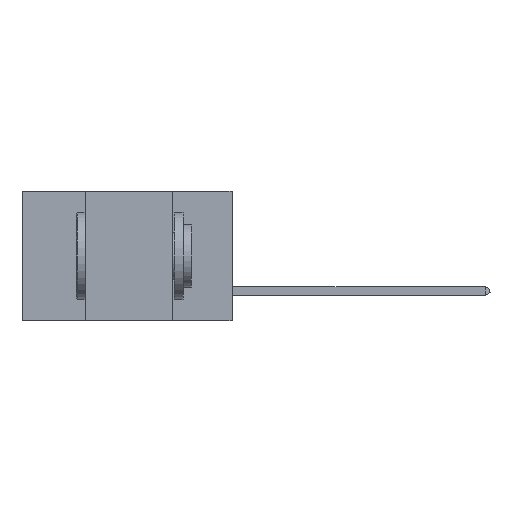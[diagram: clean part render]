
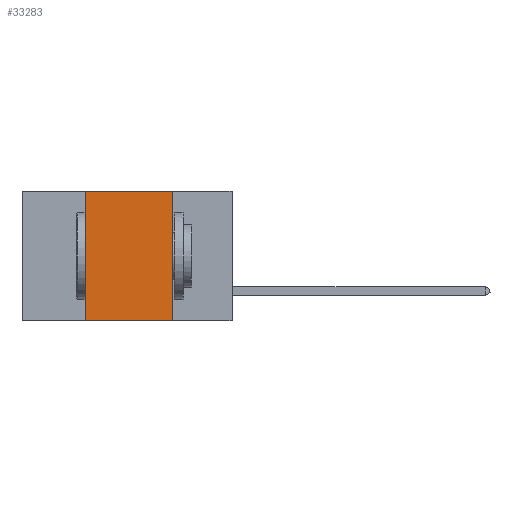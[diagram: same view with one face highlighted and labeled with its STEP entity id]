
A CAD part, left-side view. The second image highlights one B-rep face of the part: STEP entity #33283.
In plain terms, the highlighted planar face has unit normal (-1, 0, 0).
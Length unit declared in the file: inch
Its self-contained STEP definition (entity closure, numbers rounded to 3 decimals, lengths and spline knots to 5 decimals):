
#28 = VERTEX_POINT ( 'NONE', #24988 ) ;
#53 = ORIENTED_EDGE ( 'NONE', *, *, #757, .F. ) ;
#757 = EDGE_CURVE ( 'NONE', #8584, #9628, #33782, .T. ) ;
#4988 = PLANE ( 'NONE',  #29335 ) ;
#8259 = CARTESIAN_POINT ( 'NONE',  ( 0., 0.6, 0. ) ) ;
#8584 = VERTEX_POINT ( 'NONE', #9496 ) ;
#9496 = CARTESIAN_POINT ( 'NONE',  ( 0., 0.42, -0.37 ) ) ;
#9628 = VERTEX_POINT ( 'NONE', #25526 ) ;
#9767 = LINE ( 'NONE', #38687, #16532 ) ;
#12435 = ORIENTED_EDGE ( 'NONE', *, *, #34572, .F. ) ;
#12849 = DIRECTION ( 'NONE',  ( 0., 0., -1. ) ) ;
#13014 = CARTESIAN_POINT ( 'NONE',  ( 0., 0.17, 0. ) ) ;
#13269 = FACE_OUTER_BOUND ( 'NONE', #18787, .T. ) ;
#14413 = VERTEX_POINT ( 'NONE', #37573 ) ;
#15371 = DIRECTION ( 'NONE',  ( 0., 0., -1. ) ) ;
#16532 = VECTOR ( 'NONE', #31759, 39.37008 ) ;
#18787 = EDGE_LOOP ( 'NONE', ( #12435, #20275, #53, #26285 ) ) ;
#19297 = VECTOR ( 'NONE', #12849, 39.37008 ) ;
#20275 = ORIENTED_EDGE ( 'NONE', *, *, #34656, .F. ) ;
#20495 = VECTOR ( 'NONE', #46032, 39.37008 ) ;
#24217 = DIRECTION ( 'NONE',  ( 0., 0., 1. ) ) ;
#24888 = LINE ( 'NONE', #13014, #19297 ) ;
#24988 = CARTESIAN_POINT ( 'NONE',  ( 0., 0.17, 0. ) ) ;
#25526 = CARTESIAN_POINT ( 'NONE',  ( 0., 0.42, 0. ) ) ;
#26285 = ORIENTED_EDGE ( 'NONE', *, *, #29632, .T. ) ;
#29300 = VECTOR ( 'NONE', #24217, 39.37008 ) ;
#29335 = AXIS2_PLACEMENT_3D ( 'NONE', #8259, #33184, #15371 ) ;
#29632 = EDGE_CURVE ( 'NONE', #8584, #14413, #41206, .T. ) ;
#30983 = CARTESIAN_POINT ( 'NONE',  ( 0., 0.42, 0. ) ) ;
#31759 = DIRECTION ( 'NONE',  ( 0., -1., 0. ) ) ;
#32036 = CARTESIAN_POINT ( 'NONE',  ( 0., 0.6, -0.37 ) ) ;
#33184 = DIRECTION ( 'NONE',  ( 1., 0., 0. ) ) ;
#33283 = ADVANCED_FACE ( 'NONE', ( #13269 ), #4988, .F. ) ;
#33782 = LINE ( 'NONE', #30983, #29300 ) ;
#34572 = EDGE_CURVE ( 'NONE', #28, #14413, #24888, .T. ) ;
#34656 = EDGE_CURVE ( 'NONE', #9628, #28, #9767, .T. ) ;
#37573 = CARTESIAN_POINT ( 'NONE',  ( 0., 0.17, -0.37 ) ) ;
#38687 = CARTESIAN_POINT ( 'NONE',  ( 0., 0.6, 0. ) ) ;
#41206 = LINE ( 'NONE', #32036, #20495 ) ;
#46032 = DIRECTION ( 'NONE',  ( 0., -1., 0. ) ) ;
